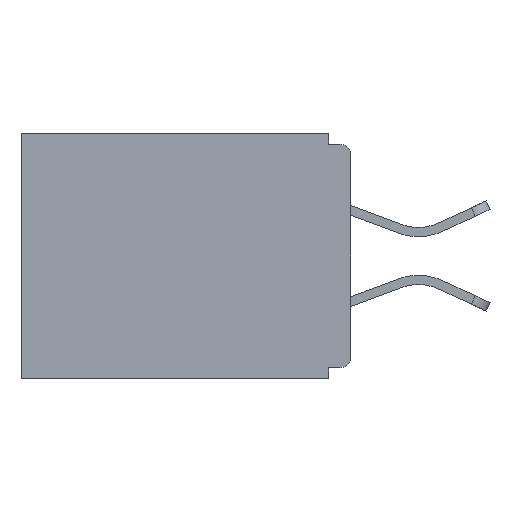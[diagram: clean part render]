
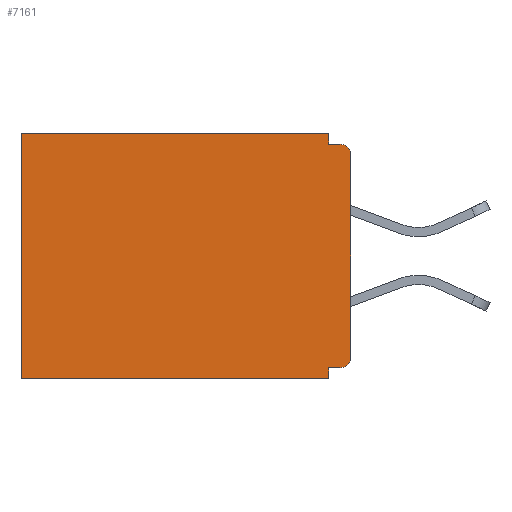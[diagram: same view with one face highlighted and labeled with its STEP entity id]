
A CAD part, left-side view. The second image highlights one B-rep face of the part: STEP entity #7161.
In plain terms, the highlighted planar face has unit normal (-1, 0, 0).
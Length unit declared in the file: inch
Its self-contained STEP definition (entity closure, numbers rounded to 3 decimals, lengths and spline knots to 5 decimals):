
#536 = CARTESIAN_POINT ( 'NONE',  ( 0.298, 0., -0.328 ) ) ;
#603 = DIRECTION ( 'NONE',  ( 0., 0., -1. ) ) ;
#704 = ORIENTED_EDGE ( 'NONE', *, *, #12481, .T. ) ;
#855 = ORIENTED_EDGE ( 'NONE', *, *, #1793, .T. ) ;
#997 = AXIS2_PLACEMENT_3D ( 'NONE', #2566, #7589, #4672 ) ;
#1022 = CARTESIAN_POINT ( 'NONE',  ( 0.298, 0.031, 0. ) ) ;
#1110 = CARTESIAN_POINT ( 'NONE',  ( 0.298, 0.031, -0.015 ) ) ;
#1202 = DIRECTION ( 'NONE',  ( 0., 0., -1. ) ) ;
#1207 = CARTESIAN_POINT ( 'NONE',  ( 0.298, 0.015, -0.03 ) ) ;
#1287 = DIRECTION ( 'NONE',  ( -1., 0., 0. ) ) ;
#1466 = VECTOR ( 'NONE', #12620, 39.37008 ) ;
#1561 = CARTESIAN_POINT ( 'NONE',  ( 0.298, 0.031, -0.343 ) ) ;
#1583 = CARTESIAN_POINT ( 'NONE',  ( 0.298, 0.46, -0.343 ) ) ;
#1793 = EDGE_CURVE ( 'NONE', #9253, #11948, #5517, .T. ) ;
#2069 = CARTESIAN_POINT ( 'NONE',  ( 0.298, 0.031, -0.328 ) ) ;
#2080 = DIRECTION ( 'NONE',  ( 0., 1., 0. ) ) ;
#2097 = ORIENTED_EDGE ( 'NONE', *, *, #3473, .F. ) ;
#2168 = LINE ( 'NONE', #10047, #5587 ) ;
#2343 = VECTOR ( 'NONE', #11344, 39.37008 ) ;
#2378 = VERTEX_POINT ( 'NONE', #7054 ) ;
#2566 = CARTESIAN_POINT ( 'NONE',  ( 0.298, 0., 0. ) ) ;
#2801 = VECTOR ( 'NONE', #11390, 39.37008 ) ;
#3074 = CIRCLE ( 'NONE', #6668, 0.015 ) ;
#3188 = EDGE_CURVE ( 'NONE', #2378, #4798, #8474, .T. ) ;
#3197 = VECTOR ( 'NONE', #2080, 39.37008 ) ;
#3460 = DIRECTION ( 'NONE',  ( 0., 1., 0. ) ) ;
#3473 = EDGE_CURVE ( 'NONE', #4798, #9760, #7362, .T. ) ;
#3590 = CARTESIAN_POINT ( 'NONE',  ( 0.298, 0., -0.343 ) ) ;
#4060 = LINE ( 'NONE', #3590, #2343 ) ;
#4079 = ORIENTED_EDGE ( 'NONE', *, *, #5903, .F. ) ;
#4177 = VERTEX_POINT ( 'NONE', #10818 ) ;
#4500 = CARTESIAN_POINT ( 'NONE',  ( 0.298, 0.015, -0.313 ) ) ;
#4672 = DIRECTION ( 'NONE',  ( 0., 0., -1. ) ) ;
#4798 = VERTEX_POINT ( 'NONE', #2069 ) ;
#5167 = DIRECTION ( 'NONE',  ( 0., 0., -1. ) ) ;
#5485 = EDGE_CURVE ( 'NONE', #11894, #10774, #8989, .T. ) ;
#5517 = LINE ( 'NONE', #10000, #3197 ) ;
#5587 = VECTOR ( 'NONE', #5167, 39.37008 ) ;
#5654 = PLANE ( 'NONE',  #997 ) ;
#5870 = CARTESIAN_POINT ( 'NONE',  ( 0.298, 0.015, -0.015 ) ) ;
#5903 = EDGE_CURVE ( 'NONE', #4177, #8818, #2168, .T. ) ;
#6288 = DIRECTION ( 'NONE',  ( 0., 0., -1. ) ) ;
#6668 = AXIS2_PLACEMENT_3D ( 'NONE', #4500, #8522, #603 ) ;
#6846 = ORIENTED_EDGE ( 'NONE', *, *, #12750, .F. ) ;
#7015 = CARTESIAN_POINT ( 'NONE',  ( 0.298, 0.46, 0. ) ) ;
#7054 = CARTESIAN_POINT ( 'NONE',  ( 0.298, 0.015, -0.328 ) ) ;
#7161 = ADVANCED_FACE ( 'NONE', ( #7576 ), #5654, .F. ) ;
#7362 = LINE ( 'NONE', #12669, #1466 ) ;
#7576 = FACE_OUTER_BOUND ( 'NONE', #7931, .T. ) ;
#7589 = DIRECTION ( 'NONE',  ( 1., 0., 0. ) ) ;
#7682 = ORIENTED_EDGE ( 'NONE', *, *, #11930, .T. ) ;
#7894 = EDGE_CURVE ( 'NONE', #2378, #8818, #3074, .T. ) ;
#7931 = EDGE_LOOP ( 'NONE', ( #704, #9002, #8595, #855, #7682, #6846, #2097, #11841, #12086, #4079 ) ) ;
#8069 = LINE ( 'NONE', #12072, #8514 ) ;
#8215 = LINE ( 'NONE', #7015, #10798 ) ;
#8474 = LINE ( 'NONE', #536, #12430 ) ;
#8514 = VECTOR ( 'NONE', #1202, 39.37008 ) ;
#8522 = DIRECTION ( 'NONE',  ( -1., 0., 0. ) ) ;
#8595 = ORIENTED_EDGE ( 'NONE', *, *, #12549, .F. ) ;
#8727 = VERTEX_POINT ( 'NONE', #1583 ) ;
#8818 = VERTEX_POINT ( 'NONE', #11595 ) ;
#8989 = LINE ( 'NONE', #10401, #2801 ) ;
#9002 = ORIENTED_EDGE ( 'NONE', *, *, #5485, .F. ) ;
#9253 = VERTEX_POINT ( 'NONE', #1022 ) ;
#9275 = CIRCLE ( 'NONE', #12094, 0.015 ) ;
#9760 = VERTEX_POINT ( 'NONE', #1561 ) ;
#9908 = CARTESIAN_POINT ( 'NONE',  ( 0.298, 0.46, 0. ) ) ;
#10000 = CARTESIAN_POINT ( 'NONE',  ( 0.298, 0., 0. ) ) ;
#10047 = CARTESIAN_POINT ( 'NONE',  ( 0.298, 0., 0. ) ) ;
#10401 = CARTESIAN_POINT ( 'NONE',  ( 0.298, 0., -0.015 ) ) ;
#10774 = VERTEX_POINT ( 'NONE', #5870 ) ;
#10798 = VECTOR ( 'NONE', #11784, 39.37008 ) ;
#10818 = CARTESIAN_POINT ( 'NONE',  ( 0.298, 0., -0.03 ) ) ;
#11344 = DIRECTION ( 'NONE',  ( 0., 1., 0. ) ) ;
#11390 = DIRECTION ( 'NONE',  ( 0., -1., 0. ) ) ;
#11595 = CARTESIAN_POINT ( 'NONE',  ( 0.298, 0., -0.313 ) ) ;
#11784 = DIRECTION ( 'NONE',  ( 0., 0., -1. ) ) ;
#11841 = ORIENTED_EDGE ( 'NONE', *, *, #3188, .F. ) ;
#11894 = VERTEX_POINT ( 'NONE', #1110 ) ;
#11930 = EDGE_CURVE ( 'NONE', #11948, #8727, #8215, .T. ) ;
#11948 = VERTEX_POINT ( 'NONE', #9908 ) ;
#12072 = CARTESIAN_POINT ( 'NONE',  ( 0.298, 0.031, -0.343 ) ) ;
#12086 = ORIENTED_EDGE ( 'NONE', *, *, #7894, .T. ) ;
#12094 = AXIS2_PLACEMENT_3D ( 'NONE', #1207, #1287, #6288 ) ;
#12430 = VECTOR ( 'NONE', #3460, 39.37008 ) ;
#12481 = EDGE_CURVE ( 'NONE', #4177, #10774, #9275, .T. ) ;
#12549 = EDGE_CURVE ( 'NONE', #9253, #11894, #8069, .T. ) ;
#12620 = DIRECTION ( 'NONE',  ( 0., 0., -1. ) ) ;
#12669 = CARTESIAN_POINT ( 'NONE',  ( 0.298, 0.031, -0.343 ) ) ;
#12750 = EDGE_CURVE ( 'NONE', #9760, #8727, #4060, .T. ) ;
